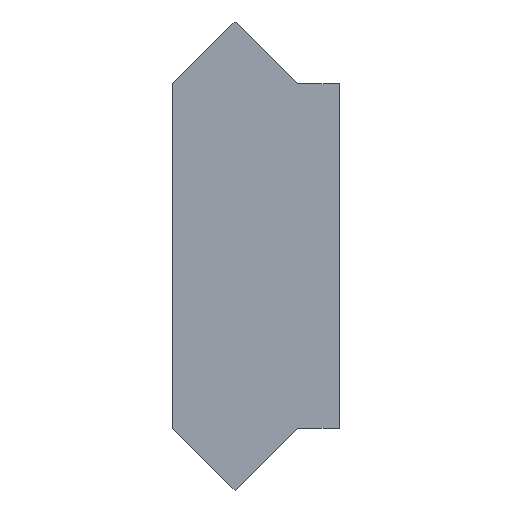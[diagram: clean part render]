
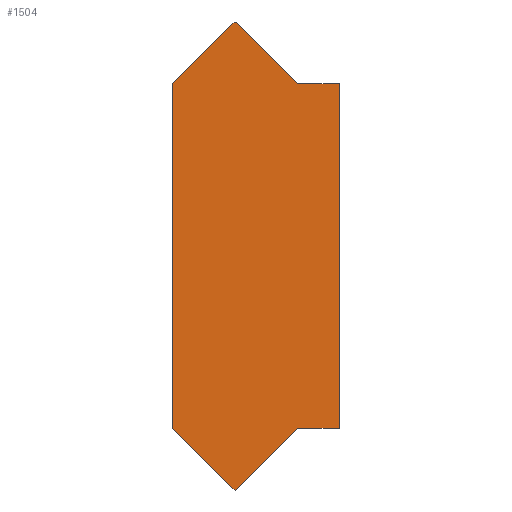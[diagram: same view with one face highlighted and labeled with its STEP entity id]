
A CAD part, left-side view. The second image highlights one B-rep face of the part: STEP entity #1504.
In plain terms, the highlighted planar face has unit normal (-1, 0, 0).
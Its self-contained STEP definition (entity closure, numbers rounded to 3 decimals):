
#48 = CARTESIAN_POINT ( 'NONE',  ( 12.7, 68.204, -8.112 ) ) ;
#78 = DIRECTION ( 'NONE',  ( 0., 0.71, 0.704 ) ) ;
#87 = VECTOR ( 'NONE', #1270, 1000. ) ;
#120 = LINE ( 'NONE', #1154, #381 ) ;
#141 = CARTESIAN_POINT ( 'NONE',  ( 12.7, 66.227, 8.113 ) ) ;
#144 = VECTOR ( 'NONE', #957, 1000. ) ;
#153 = VERTEX_POINT ( 'NONE', #141 ) ;
#160 = CARTESIAN_POINT ( 'NONE',  ( 12.7, 74.084, -8.113 ) ) ;
#194 = AXIS2_PLACEMENT_3D ( 'NONE', #529, #1468, #1605 ) ;
#229 = ORIENTED_EDGE ( 'NONE', *, *, #1725, .F. ) ;
#266 = EDGE_CURVE ( 'NONE', #1423, #607, #120, .T. ) ;
#281 = VECTOR ( 'NONE', #588, 1000. ) ;
#333 = LINE ( 'NONE', #576, #1364 ) ;
#356 = LINE ( 'NONE', #643, #456 ) ;
#358 = LINE ( 'NONE', #582, #281 ) ;
#362 = EDGE_CURVE ( 'NONE', #153, #718, #1059, .T. ) ;
#381 = VECTOR ( 'NONE', #1285, 1000. ) ;
#456 = VECTOR ( 'NONE', #1036, 1000. ) ;
#460 = EDGE_CURVE ( 'NONE', #1329, #718, #333, .T. ) ;
#508 = CARTESIAN_POINT ( 'NONE',  ( 12.7, 71.145, -11.025 ) ) ;
#517 = CARTESIAN_POINT ( 'NONE',  ( 12.7, 66.86, 6.78 ) ) ;
#529 = CARTESIAN_POINT ( 'NONE',  ( 12.7, 38.962, -18.5 ) ) ;
#531 = VERTEX_POINT ( 'NONE', #835 ) ;
#540 = ORIENTED_EDGE ( 'NONE', *, *, #266, .F. ) ;
#576 = CARTESIAN_POINT ( 'NONE',  ( 12.7, 68.127, -8.112 ) ) ;
#582 = CARTESIAN_POINT ( 'NONE',  ( 12.7, 62.999, 8.113 ) ) ;
#588 = DIRECTION ( 'NONE',  ( 0., 1., 0. ) ) ;
#607 = VERTEX_POINT ( 'NONE', #1382 ) ;
#634 = FACE_OUTER_BOUND ( 'NONE', #890, .T. ) ;
#643 = CARTESIAN_POINT ( 'NONE',  ( 12.7, 70.568, 11.596 ) ) ;
#664 = DIRECTION ( 'NONE',  ( 0., -0.71, -0.704 ) ) ;
#718 = VERTEX_POINT ( 'NONE', #1733 ) ;
#739 = ORIENTED_EDGE ( 'NONE', *, *, #1165, .F. ) ;
#740 = CARTESIAN_POINT ( 'NONE',  ( 12.7, 68.204, 8.113 ) ) ;
#755 = VERTEX_POINT ( 'NONE', #508 ) ;
#760 = EDGE_CURVE ( 'NONE', #531, #997, #989, .T. ) ;
#835 = CARTESIAN_POINT ( 'NONE',  ( 12.7, 71.145, 11.025 ) ) ;
#890 = EDGE_LOOP ( 'NONE', ( #1038, #922, #1039, #739, #540, #1212, #229, #1175 ) ) ;
#902 = LINE ( 'NONE', #1118, #87 ) ;
#922 = ORIENTED_EDGE ( 'NONE', *, *, #1539, .T. ) ;
#932 = VECTOR ( 'NONE', #664, 1000. ) ;
#957 = DIRECTION ( 'NONE',  ( 0., 0., -1. ) ) ;
#989 = LINE ( 'NONE', #517, #932 ) ;
#997 = VERTEX_POINT ( 'NONE', #740 ) ;
#1004 = CARTESIAN_POINT ( 'NONE',  ( 12.7, 66.227, -23.578 ) ) ;
#1036 = DIRECTION ( 'NONE',  ( 0., -0.71, 0.704 ) ) ;
#1038 = ORIENTED_EDGE ( 'NONE', *, *, #362, .F. ) ;
#1039 = ORIENTED_EDGE ( 'NONE', *, *, #760, .F. ) ;
#1059 = LINE ( 'NONE', #1004, #144 ) ;
#1060 = PLANE ( 'NONE',  #194 ) ;
#1118 = CARTESIAN_POINT ( 'NONE',  ( 12.7, 68.097, -8.006 ) ) ;
#1154 = CARTESIAN_POINT ( 'NONE',  ( 12.7, 74.084, -5.425 ) ) ;
#1165 = EDGE_CURVE ( 'NONE', #607, #531, #356, .T. ) ;
#1175 = ORIENTED_EDGE ( 'NONE', *, *, #460, .T. ) ;
#1212 = ORIENTED_EDGE ( 'NONE', *, *, #1689, .F. ) ;
#1270 = DIRECTION ( 'NONE',  ( 0., 0.71, -0.704 ) ) ;
#1285 = DIRECTION ( 'NONE',  ( 0., 0., 1. ) ) ;
#1329 = VERTEX_POINT ( 'NONE', #48 ) ;
#1364 = VECTOR ( 'NONE', #1521, 1000. ) ;
#1382 = CARTESIAN_POINT ( 'NONE',  ( 12.7, 74.084, 8.113 ) ) ;
#1404 = CARTESIAN_POINT ( 'NONE',  ( 12.7, 62.788, -19.303 ) ) ;
#1423 = VERTEX_POINT ( 'NONE', #160 ) ;
#1468 = DIRECTION ( 'NONE',  ( -1., 0., 0. ) ) ;
#1504 = ADVANCED_FACE ( 'NONE', ( #634 ), #1060, .T. ) ;
#1521 = DIRECTION ( 'NONE',  ( 0., -1., 0. ) ) ;
#1539 = EDGE_CURVE ( 'NONE', #153, #997, #358, .T. ) ;
#1605 = DIRECTION ( 'NONE',  ( 0., 0., -1. ) ) ;
#1654 = VECTOR ( 'NONE', #78, 1000. ) ;
#1689 = EDGE_CURVE ( 'NONE', #755, #1423, #1699, .T. ) ;
#1699 = LINE ( 'NONE', #1404, #1654 ) ;
#1725 = EDGE_CURVE ( 'NONE', #1329, #755, #902, .T. ) ;
#1733 = CARTESIAN_POINT ( 'NONE',  ( 12.7, 66.227, -8.112 ) ) ;
